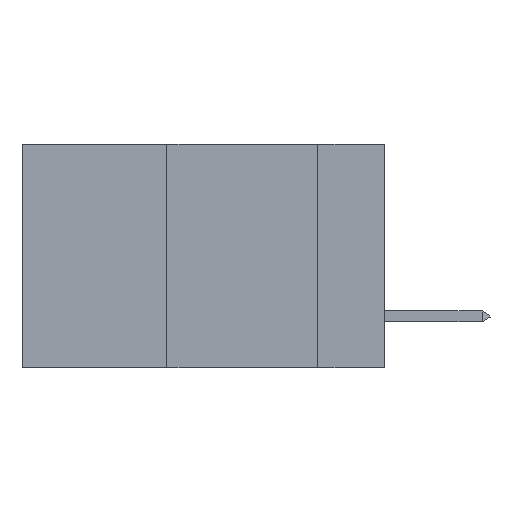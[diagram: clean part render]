
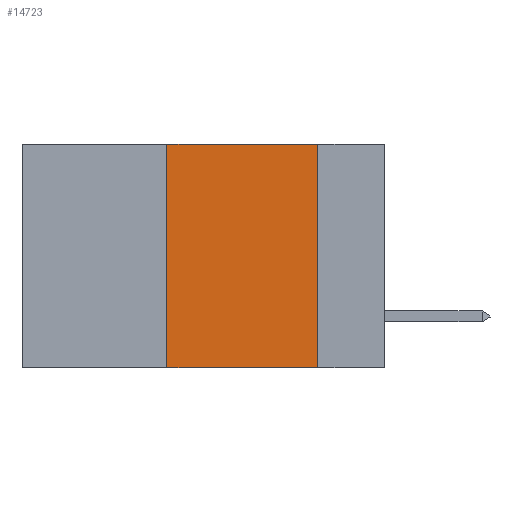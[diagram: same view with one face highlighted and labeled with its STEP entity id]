
A CAD part, left-side view. The second image highlights one B-rep face of the part: STEP entity #14723.
In plain terms, the highlighted planar face has unit normal (-1, 0, 0).
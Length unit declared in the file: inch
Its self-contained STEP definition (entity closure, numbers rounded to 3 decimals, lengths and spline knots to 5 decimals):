
#2671 = CARTESIAN_POINT ( 'NONE',  ( 0., 0.6, 0. ) ) ;
#4118 = ORIENTED_EDGE ( 'NONE', *, *, #5477, .T. ) ;
#5477 = EDGE_CURVE ( 'NONE', #45073, #32422, #36232, .T. ) ;
#5552 = CARTESIAN_POINT ( 'NONE',  ( 0., 0.11, 0. ) ) ;
#5594 = DIRECTION ( 'NONE',  ( 1., 0., 0. ) ) ;
#6146 = LINE ( 'NONE', #5552, #14469 ) ;
#6273 = EDGE_CURVE ( 'NONE', #28045, #32422, #6146, .T. ) ;
#7845 = VECTOR ( 'NONE', #10063, 39.37008 ) ;
#9316 = PLANE ( 'NONE',  #27638 ) ;
#10063 = DIRECTION ( 'NONE',  ( 0., -1., 0. ) ) ;
#14469 = VECTOR ( 'NONE', #19819, 39.37008 ) ;
#14723 = ADVANCED_FACE ( 'NONE', ( #40379 ), #9316, .F. ) ;
#17832 = LINE ( 'NONE', #45219, #7845 ) ;
#19502 = ORIENTED_EDGE ( 'NONE', *, *, #29819, .F. ) ;
#19819 = DIRECTION ( 'NONE',  ( 0., 0., -1. ) ) ;
#20031 = DIRECTION ( 'NONE',  ( 0., 0., -1. ) ) ;
#20213 = ORIENTED_EDGE ( 'NONE', *, *, #6273, .F. ) ;
#20964 = DIRECTION ( 'NONE',  ( 0., -1., 0. ) ) ;
#21539 = CARTESIAN_POINT ( 'NONE',  ( 0., 0.6, -0.37 ) ) ;
#21672 = EDGE_LOOP ( 'NONE', ( #20213, #19502, #28859, #4118 ) ) ;
#27638 = AXIS2_PLACEMENT_3D ( 'NONE', #2671, #5594, #20031 ) ;
#27927 = LINE ( 'NONE', #39131, #28437 ) ;
#28045 = VERTEX_POINT ( 'NONE', #42909 ) ;
#28437 = VECTOR ( 'NONE', #36105, 39.37008 ) ;
#28859 = ORIENTED_EDGE ( 'NONE', *, *, #40456, .F. ) ;
#29717 = VERTEX_POINT ( 'NONE', #45514 ) ;
#29819 = EDGE_CURVE ( 'NONE', #29717, #28045, #17832, .T. ) ;
#32200 = CARTESIAN_POINT ( 'NONE',  ( 0., 0.11, -0.37 ) ) ;
#32422 = VERTEX_POINT ( 'NONE', #32200 ) ;
#36105 = DIRECTION ( 'NONE',  ( 0., 0., 1. ) ) ;
#36232 = LINE ( 'NONE', #21539, #40740 ) ;
#39131 = CARTESIAN_POINT ( 'NONE',  ( 0., 0.36, 0. ) ) ;
#40379 = FACE_OUTER_BOUND ( 'NONE', #21672, .T. ) ;
#40456 = EDGE_CURVE ( 'NONE', #45073, #29717, #27927, .T. ) ;
#40740 = VECTOR ( 'NONE', #20964, 39.37008 ) ;
#42909 = CARTESIAN_POINT ( 'NONE',  ( 0., 0.11, 0. ) ) ;
#43517 = CARTESIAN_POINT ( 'NONE',  ( 0., 0.36, -0.37 ) ) ;
#45073 = VERTEX_POINT ( 'NONE', #43517 ) ;
#45219 = CARTESIAN_POINT ( 'NONE',  ( 0., 0.6, 0. ) ) ;
#45514 = CARTESIAN_POINT ( 'NONE',  ( 0., 0.36, 0. ) ) ;
